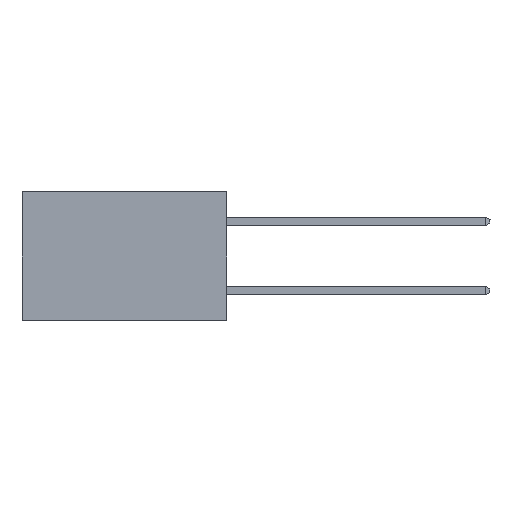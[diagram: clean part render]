
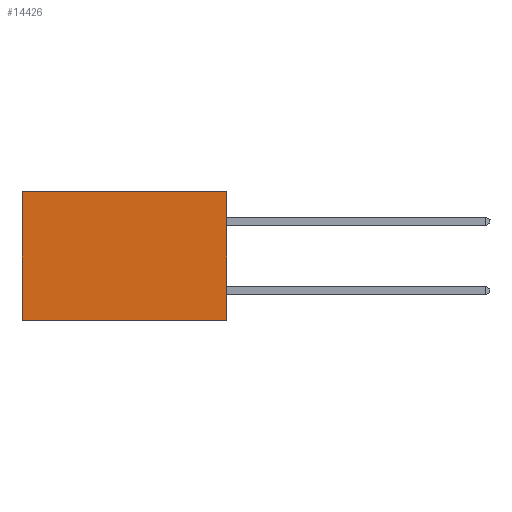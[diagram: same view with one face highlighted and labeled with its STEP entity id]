
A CAD part, left-side view. The second image highlights one B-rep face of the part: STEP entity #14426.
In plain terms, the highlighted planar face has unit normal (-1, 0, 0).
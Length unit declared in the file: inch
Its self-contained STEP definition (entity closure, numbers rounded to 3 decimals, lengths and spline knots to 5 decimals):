
#245 = CARTESIAN_POINT ( 'NONE',  ( 0.277, 0., 0. ) ) ;
#1662 = VERTEX_POINT ( 'NONE', #17063 ) ;
#1765 = VECTOR ( 'NONE', #14943, 39.37008 ) ;
#3169 = CARTESIAN_POINT ( 'NONE',  ( 0.277, 0., -0.37 ) ) ;
#3227 = DIRECTION ( 'NONE',  ( 1., 0., 0. ) ) ;
#3539 = AXIS2_PLACEMENT_3D ( 'NONE', #14716, #3227, #16625 ) ;
#5294 = VERTEX_POINT ( 'NONE', #245 ) ;
#5423 = DIRECTION ( 'NONE',  ( 0., 1., 0. ) ) ;
#5435 = EDGE_CURVE ( 'NONE', #5294, #1662, #16281, .T. ) ;
#6197 = VECTOR ( 'NONE', #19296, 39.37008 ) ;
#7172 = VECTOR ( 'NONE', #5423, 39.37008 ) ;
#7783 = LINE ( 'NONE', #14910, #7172 ) ;
#7917 = ORIENTED_EDGE ( 'NONE', *, *, #10547, .F. ) ;
#8381 = LINE ( 'NONE', #16643, #22722 ) ;
#10513 = EDGE_CURVE ( 'NONE', #1662, #17223, #8381, .T. ) ;
#10547 = EDGE_CURVE ( 'NONE', #13711, #17223, #7783, .T. ) ;
#10877 = CARTESIAN_POINT ( 'NONE',  ( 0.277, 0.59, -0.37 ) ) ;
#11193 = CARTESIAN_POINT ( 'NONE',  ( 0.277, 0., -0.37 ) ) ;
#13126 = EDGE_CURVE ( 'NONE', #5294, #13711, #22009, .T. ) ;
#13711 = VERTEX_POINT ( 'NONE', #3169 ) ;
#14281 = EDGE_LOOP ( 'NONE', ( #16764, #7917, #14694, #22577 ) ) ;
#14426 = ADVANCED_FACE ( 'NONE', ( #18161 ), #23986, .F. ) ;
#14694 = ORIENTED_EDGE ( 'NONE', *, *, #13126, .F. ) ;
#14716 = CARTESIAN_POINT ( 'NONE',  ( 0.277, 0., -0.37 ) ) ;
#14910 = CARTESIAN_POINT ( 'NONE',  ( 0.277, 0., -0.37 ) ) ;
#14943 = DIRECTION ( 'NONE',  ( 0., 0., -1. ) ) ;
#16281 = LINE ( 'NONE', #19267, #6197 ) ;
#16625 = DIRECTION ( 'NONE',  ( 0., 0., -1. ) ) ;
#16643 = CARTESIAN_POINT ( 'NONE',  ( 0.277, 0.59, -0.37 ) ) ;
#16764 = ORIENTED_EDGE ( 'NONE', *, *, #10513, .T. ) ;
#17063 = CARTESIAN_POINT ( 'NONE',  ( 0.277, 0.59, 0. ) ) ;
#17223 = VERTEX_POINT ( 'NONE', #10877 ) ;
#18161 = FACE_OUTER_BOUND ( 'NONE', #14281, .T. ) ;
#19267 = CARTESIAN_POINT ( 'NONE',  ( 0.277, 0., 0. ) ) ;
#19296 = DIRECTION ( 'NONE',  ( 0., 1., 0. ) ) ;
#22009 = LINE ( 'NONE', #11193, #1765 ) ;
#22244 = DIRECTION ( 'NONE',  ( 0., 0., -1. ) ) ;
#22577 = ORIENTED_EDGE ( 'NONE', *, *, #5435, .T. ) ;
#22722 = VECTOR ( 'NONE', #22244, 39.37008 ) ;
#23986 = PLANE ( 'NONE',  #3539 ) ;
